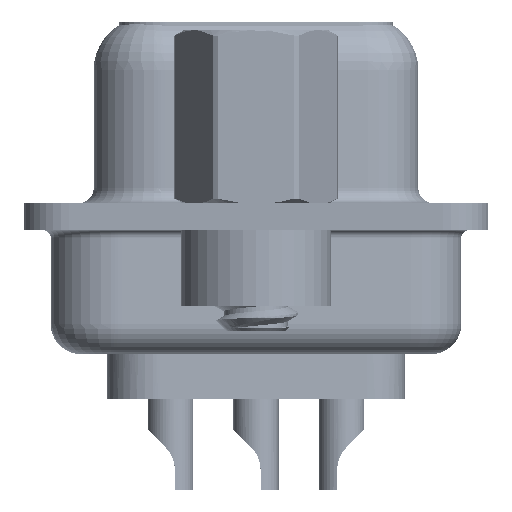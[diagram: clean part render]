
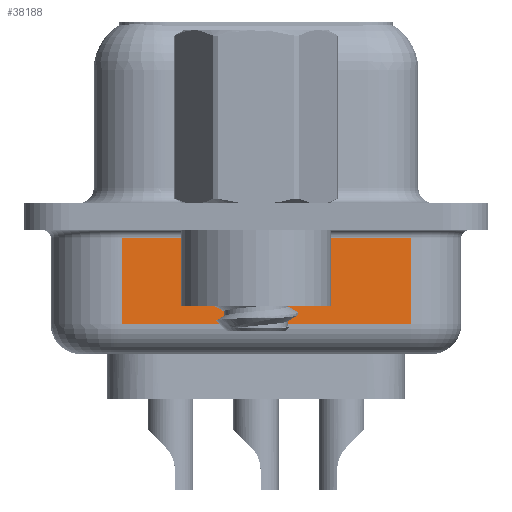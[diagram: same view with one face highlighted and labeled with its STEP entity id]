
A CAD part, left-side view. The second image highlights one B-rep face of the part: STEP entity #38188.
In plain terms, the highlighted planar face has unit normal (-0.985, -0.174, 0).
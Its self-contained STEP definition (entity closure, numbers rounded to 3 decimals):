
#1191 = VERTEX_POINT ( 'NONE', #41831 ) ;
#2252 = CARTESIAN_POINT ( 'NONE',  ( 2.93, 4.453, -3.55 ) ) ;
#2819 = DIRECTION ( 'NONE',  ( -0.174, 0.985, 0. ) ) ;
#6021 = VECTOR ( 'NONE', #38736, 1000. ) ;
#6298 = DIRECTION ( 'NONE',  ( 0.985, 0.174, 0. ) ) ;
#6650 = AXIS2_PLACEMENT_3D ( 'NONE', #32599, #6298, #2819 ) ;
#7332 = VERTEX_POINT ( 'NONE', #11996 ) ;
#7849 = LINE ( 'NONE', #21777, #23363 ) ;
#8982 = EDGE_CURVE ( 'NONE', #7332, #1191, #7849, .T. ) ;
#9158 = LINE ( 'NONE', #12220, #6021 ) ;
#10144 = CARTESIAN_POINT ( 'NONE',  ( 2.93, 4.453, -0.7 ) ) ;
#10360 = ORIENTED_EDGE ( 'NONE', *, *, #18042, .F. ) ;
#11323 = DIRECTION ( 'NONE',  ( 0., 0., 1. ) ) ;
#11643 = EDGE_CURVE ( 'NONE', #14317, #7332, #37895, .T. ) ;
#11942 = CARTESIAN_POINT ( 'NONE',  ( 2.93, 4.453, -0.7 ) ) ;
#11996 = CARTESIAN_POINT ( 'NONE',  ( 4.623, -5.147, -3.55 ) ) ;
#12220 = CARTESIAN_POINT ( 'NONE',  ( 2.93, 4.453, -4.55 ) ) ;
#14317 = VERTEX_POINT ( 'NONE', #2252 ) ;
#15197 = EDGE_CURVE ( 'NONE', #1191, #26944, #22587, .T. ) ;
#18042 = EDGE_CURVE ( 'NONE', #14317, #26944, #9158, .T. ) ;
#21187 = CARTESIAN_POINT ( 'NONE',  ( 2.93, 4.453, -3.55 ) ) ;
#21777 = CARTESIAN_POINT ( 'NONE',  ( 4.623, -5.147, -4.55 ) ) ;
#22587 = LINE ( 'NONE', #11942, #22999 ) ;
#22613 = EDGE_LOOP ( 'NONE', ( #10360, #23377, #33311, #24705 ) ) ;
#22999 = VECTOR ( 'NONE', #35833, 1000. ) ;
#23363 = VECTOR ( 'NONE', #11323, 1000. ) ;
#23377 = ORIENTED_EDGE ( 'NONE', *, *, #11643, .T. ) ;
#24705 = ORIENTED_EDGE ( 'NONE', *, *, #15197, .T. ) ;
#26944 = VERTEX_POINT ( 'NONE', #10144 ) ;
#32599 = CARTESIAN_POINT ( 'NONE',  ( 2.93, 4.453, -4.55 ) ) ;
#33311 = ORIENTED_EDGE ( 'NONE', *, *, #8982, .T. ) ;
#34430 = DIRECTION ( 'NONE',  ( 0.174, -0.985, 0. ) ) ;
#35833 = DIRECTION ( 'NONE',  ( -0.174, 0.985, 0. ) ) ;
#37895 = LINE ( 'NONE', #21187, #38724 ) ;
#38188 = ADVANCED_FACE ( 'NONE', ( #40171 ), #39323, .F. ) ;
#38724 = VECTOR ( 'NONE', #34430, 1000. ) ;
#38736 = DIRECTION ( 'NONE',  ( 0., 0., 1. ) ) ;
#39323 = PLANE ( 'NONE',  #6650 ) ;
#40171 = FACE_OUTER_BOUND ( 'NONE', #22613, .T. ) ;
#41831 = CARTESIAN_POINT ( 'NONE',  ( 4.623, -5.147, -0.7 ) ) ;
